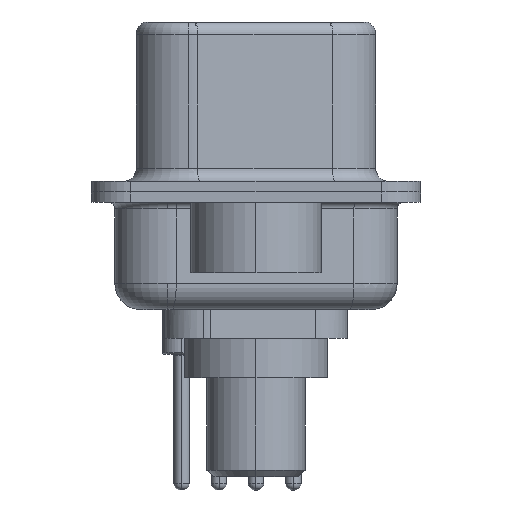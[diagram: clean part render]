
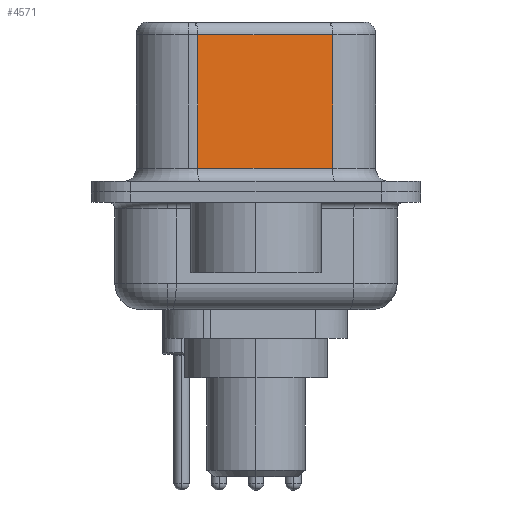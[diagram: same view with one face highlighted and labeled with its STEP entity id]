
A CAD part, left-side view. The second image highlights one B-rep face of the part: STEP entity #4571.
In plain terms, the highlighted planar face has unit normal (-0.985, -0.174, 0).
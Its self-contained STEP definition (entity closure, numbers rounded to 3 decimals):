
#98 = CARTESIAN_POINT ( 'NONE',  ( 3.67, 2.233, 6.52 ) ) ;
#3739 = FACE_OUTER_BOUND ( 'NONE', #9999, .T. ) ;
#4299 = LINE ( 'NONE', #98, #8994 ) ;
#4571 = ADVANCED_FACE ( 'NONE', ( #3739 ), #10760, .F. ) ;
#5329 = DIRECTION ( 'NONE',  ( 0., 0., -1. ) ) ;
#5948 = CARTESIAN_POINT ( 'NONE',  ( 4.58, -2.927, 6.52 ) ) ;
#6139 = ORIENTED_EDGE ( 'NONE', *, *, #13507, .T. ) ;
#7039 = DIRECTION ( 'NONE',  ( 0.174, -0.985, 0. ) ) ;
#8295 = VECTOR ( 'NONE', #7039, 1000. ) ;
#8994 = VECTOR ( 'NONE', #5329, 1000. ) ;
#9495 = CARTESIAN_POINT ( 'NONE',  ( 3.67, 2.233, 6.02 ) ) ;
#9583 = AXIS2_PLACEMENT_3D ( 'NONE', #23094, #16986, #16799 ) ;
#9999 = EDGE_LOOP ( 'NONE', ( #16534, #13950, #6139, #14445 ) ) ;
#10298 = CARTESIAN_POINT ( 'NONE',  ( 3.67, 2.233, 0.9 ) ) ;
#10760 = PLANE ( 'NONE',  #9583 ) ;
#11437 = VERTEX_POINT ( 'NONE', #10298 ) ;
#12456 = CARTESIAN_POINT ( 'NONE',  ( 4.58, -2.927, 6.02 ) ) ;
#12908 = CARTESIAN_POINT ( 'NONE',  ( 4.58, -2.927, 0.9 ) ) ;
#12952 = VERTEX_POINT ( 'NONE', #12908 ) ;
#13049 = DIRECTION ( 'NONE',  ( 0., 0., -1. ) ) ;
#13507 = EDGE_CURVE ( 'NONE', #13745, #11437, #4299, .T. ) ;
#13745 = VERTEX_POINT ( 'NONE', #9495 ) ;
#13950 = ORIENTED_EDGE ( 'NONE', *, *, #15714, .T. ) ;
#14315 = DIRECTION ( 'NONE',  ( -0.174, 0.985, 0. ) ) ;
#14445 = ORIENTED_EDGE ( 'NONE', *, *, #18945, .T. ) ;
#15714 = EDGE_CURVE ( 'NONE', #18520, #13745, #20114, .T. ) ;
#15852 = VECTOR ( 'NONE', #13049, 1000. ) ;
#16534 = ORIENTED_EDGE ( 'NONE', *, *, #22498, .F. ) ;
#16799 = DIRECTION ( 'NONE',  ( -0.174, 0.985, 0. ) ) ;
#16986 = DIRECTION ( 'NONE',  ( 0.985, 0.174, 0. ) ) ;
#17727 = CARTESIAN_POINT ( 'NONE',  ( 4.58, -2.927, 0.9 ) ) ;
#18520 = VERTEX_POINT ( 'NONE', #20060 ) ;
#18945 = EDGE_CURVE ( 'NONE', #11437, #12952, #21416, .T. ) ;
#19572 = VECTOR ( 'NONE', #14315, 1000. ) ;
#20060 = CARTESIAN_POINT ( 'NONE',  ( 4.58, -2.927, 6.02 ) ) ;
#20114 = LINE ( 'NONE', #12456, #19572 ) ;
#20544 = LINE ( 'NONE', #5948, #15852 ) ;
#21416 = LINE ( 'NONE', #17727, #8295 ) ;
#22498 = EDGE_CURVE ( 'NONE', #18520, #12952, #20544, .T. ) ;
#23094 = CARTESIAN_POINT ( 'NONE',  ( 4.58, -2.927, 6.52 ) ) ;
